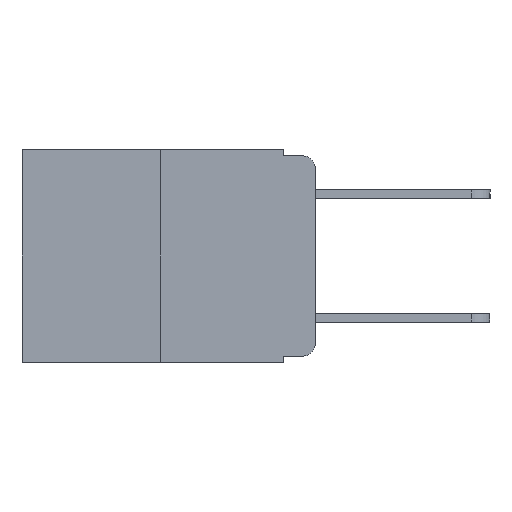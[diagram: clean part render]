
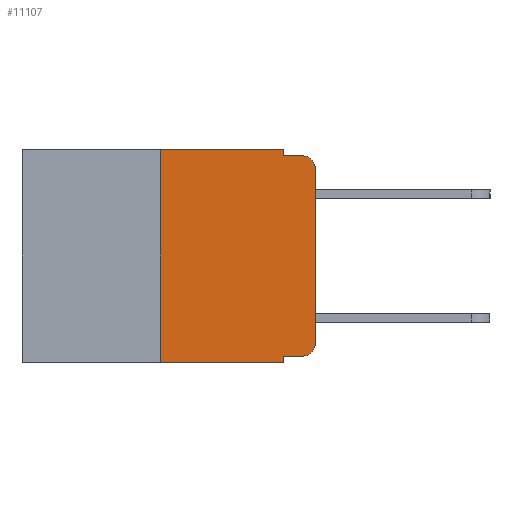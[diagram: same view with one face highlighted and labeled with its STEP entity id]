
A CAD part, left-side view. The second image highlights one B-rep face of the part: STEP entity #11107.
In plain terms, the highlighted planar face has unit normal (-1, 0, 0).
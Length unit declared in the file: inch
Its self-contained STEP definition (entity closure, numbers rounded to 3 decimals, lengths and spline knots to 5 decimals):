
#101 = VERTEX_POINT ( 'NONE', #3168 ) ;
#272 = DIRECTION ( 'NONE',  ( 0., -1., 0. ) ) ;
#390 = CIRCLE ( 'NONE', #5110, 0.02 ) ;
#718 = EDGE_CURVE ( 'NONE', #10632, #4943, #1104, .T. ) ;
#1095 = CARTESIAN_POINT ( 'NONE',  ( 0., 0.051, 0. ) ) ;
#1104 = LINE ( 'NONE', #2223, #7370 ) ;
#1519 = AXIS2_PLACEMENT_3D ( 'NONE', #3217, #9180, #4093 ) ;
#1817 = CARTESIAN_POINT ( 'NONE',  ( 0., 0., -0.313 ) ) ;
#1832 = VERTEX_POINT ( 'NONE', #10138 ) ;
#1908 = ORIENTED_EDGE ( 'NONE', *, *, #10417, .T. ) ;
#1977 = CARTESIAN_POINT ( 'NONE',  ( 0., 0.02, -0.03 ) ) ;
#2223 = CARTESIAN_POINT ( 'NONE',  ( 0., 0.473, 0. ) ) ;
#2315 = PLANE ( 'NONE',  #1519 ) ;
#2859 = VECTOR ( 'NONE', #6938, 39.37008 ) ;
#2863 = DIRECTION ( 'NONE',  ( 0., 0., -1. ) ) ;
#3168 = CARTESIAN_POINT ( 'NONE',  ( 0., 0.051, -0.343 ) ) ;
#3217 = CARTESIAN_POINT ( 'NONE',  ( 0., 0.473, 0. ) ) ;
#3360 = VECTOR ( 'NONE', #11057, 39.37008 ) ;
#3378 = VERTEX_POINT ( 'NONE', #8397 ) ;
#3407 = CARTESIAN_POINT ( 'NONE',  ( 0., 0.25, 0. ) ) ;
#3445 = VECTOR ( 'NONE', #8265, 39.37008 ) ;
#3498 = LINE ( 'NONE', #4645, #9950 ) ;
#3635 = CARTESIAN_POINT ( 'NONE',  ( 0., 0.051, 0. ) ) ;
#3728 = CARTESIAN_POINT ( 'NONE',  ( 0., 0.02, -0.333 ) ) ;
#3730 = ORIENTED_EDGE ( 'NONE', *, *, #8301, .F. ) ;
#3810 = VECTOR ( 'NONE', #6124, 39.37008 ) ;
#3885 = LINE ( 'NONE', #9499, #6285 ) ;
#3960 = CARTESIAN_POINT ( 'NONE',  ( 0., 0.051, -0.333 ) ) ;
#4093 = DIRECTION ( 'NONE',  ( 0., 0., -1. ) ) ;
#4317 = VERTEX_POINT ( 'NONE', #3728 ) ;
#4479 = DIRECTION ( 'NONE',  ( 0., -1., 0. ) ) ;
#4524 = EDGE_LOOP ( 'NONE', ( #5395, #1908, #9182, #4712, #7294, #5164, #8303, #3730, #10850, #8672 ) ) ;
#4645 = CARTESIAN_POINT ( 'NONE',  ( 0., 0., 0. ) ) ;
#4712 = ORIENTED_EDGE ( 'NONE', *, *, #10359, .F. ) ;
#4943 = VERTEX_POINT ( 'NONE', #6328 ) ;
#5110 = AXIS2_PLACEMENT_3D ( 'NONE', #6321, #6264, #6210 ) ;
#5164 = ORIENTED_EDGE ( 'NONE', *, *, #8258, .F. ) ;
#5286 = VERTEX_POINT ( 'NONE', #8650 ) ;
#5395 = ORIENTED_EDGE ( 'NONE', *, *, #10421, .T. ) ;
#5509 = LINE ( 'NONE', #1095, #2859 ) ;
#5709 = LINE ( 'NONE', #3635, #3360 ) ;
#6124 = DIRECTION ( 'NONE',  ( 0., -1., 0. ) ) ;
#6138 = CARTESIAN_POINT ( 'NONE',  ( 0., 0.473, -0.343 ) ) ;
#6210 = DIRECTION ( 'NONE',  ( 0., 0., -1. ) ) ;
#6264 = DIRECTION ( 'NONE',  ( -1., 0., 0. ) ) ;
#6285 = VECTOR ( 'NONE', #4479, 39.37008 ) ;
#6321 = CARTESIAN_POINT ( 'NONE',  ( 0., 0.02, -0.313 ) ) ;
#6328 = CARTESIAN_POINT ( 'NONE',  ( 0., 0.051, 0. ) ) ;
#6887 = DIRECTION ( 'NONE',  ( 0., -1., 0. ) ) ;
#6931 = CARTESIAN_POINT ( 'NONE',  ( 0., 0.051, -0.333 ) ) ;
#6938 = DIRECTION ( 'NONE',  ( 0., 0., -1. ) ) ;
#7294 = ORIENTED_EDGE ( 'NONE', *, *, #718, .F. ) ;
#7370 = VECTOR ( 'NONE', #272, 39.37008 ) ;
#7535 = LINE ( 'NONE', #6931, #9404 ) ;
#7747 = VERTEX_POINT ( 'NONE', #1817 ) ;
#7811 = FACE_OUTER_BOUND ( 'NONE', #4524, .T. ) ;
#7923 = AXIS2_PLACEMENT_3D ( 'NONE', #1977, #8079, #2863 ) ;
#8079 = DIRECTION ( 'NONE',  ( -1., 0., 0. ) ) ;
#8199 = VERTEX_POINT ( 'NONE', #8917 ) ;
#8258 = EDGE_CURVE ( 'NONE', #1832, #10632, #10122, .T. ) ;
#8265 = DIRECTION ( 'NONE',  ( 0., 0., 1. ) ) ;
#8301 = EDGE_CURVE ( 'NONE', #10052, #101, #5509, .T. ) ;
#8303 = ORIENTED_EDGE ( 'NONE', *, *, #8977, .T. ) ;
#8314 = EDGE_CURVE ( 'NONE', #10052, #4317, #7535, .T. ) ;
#8315 = EDGE_CURVE ( 'NONE', #4317, #7747, #390, .T. ) ;
#8372 = CARTESIAN_POINT ( 'NONE',  ( 0., 0.25, 0. ) ) ;
#8397 = CARTESIAN_POINT ( 'NONE',  ( 0., 0., -0.03 ) ) ;
#8650 = CARTESIAN_POINT ( 'NONE',  ( 0., 0.051, -0.01 ) ) ;
#8672 = ORIENTED_EDGE ( 'NONE', *, *, #8315, .T. ) ;
#8917 = CARTESIAN_POINT ( 'NONE',  ( 0., 0.02, -0.01 ) ) ;
#8977 = EDGE_CURVE ( 'NONE', #1832, #101, #10215, .T. ) ;
#9180 = DIRECTION ( 'NONE',  ( 1., 0., 0. ) ) ;
#9182 = ORIENTED_EDGE ( 'NONE', *, *, #10341, .F. ) ;
#9404 = VECTOR ( 'NONE', #6887, 39.37008 ) ;
#9499 = CARTESIAN_POINT ( 'NONE',  ( 0., 0.051, -0.01 ) ) ;
#9655 = DIRECTION ( 'NONE',  ( 0., 0., 1. ) ) ;
#9950 = VECTOR ( 'NONE', #9655, 39.37008 ) ;
#10052 = VERTEX_POINT ( 'NONE', #3960 ) ;
#10122 = LINE ( 'NONE', #3407, #3445 ) ;
#10138 = CARTESIAN_POINT ( 'NONE',  ( 0., 0.25, -0.343 ) ) ;
#10167 = CIRCLE ( 'NONE', #7923, 0.02 ) ;
#10215 = LINE ( 'NONE', #6138, #3810 ) ;
#10341 = EDGE_CURVE ( 'NONE', #5286, #8199, #3885, .T. ) ;
#10359 = EDGE_CURVE ( 'NONE', #4943, #5286, #5709, .T. ) ;
#10417 = EDGE_CURVE ( 'NONE', #3378, #8199, #10167, .T. ) ;
#10421 = EDGE_CURVE ( 'NONE', #7747, #3378, #3498, .T. ) ;
#10632 = VERTEX_POINT ( 'NONE', #8372 ) ;
#10850 = ORIENTED_EDGE ( 'NONE', *, *, #8314, .T. ) ;
#11057 = DIRECTION ( 'NONE',  ( 0., 0., -1. ) ) ;
#11107 = ADVANCED_FACE ( 'NONE', ( #7811 ), #2315, .F. ) ;
